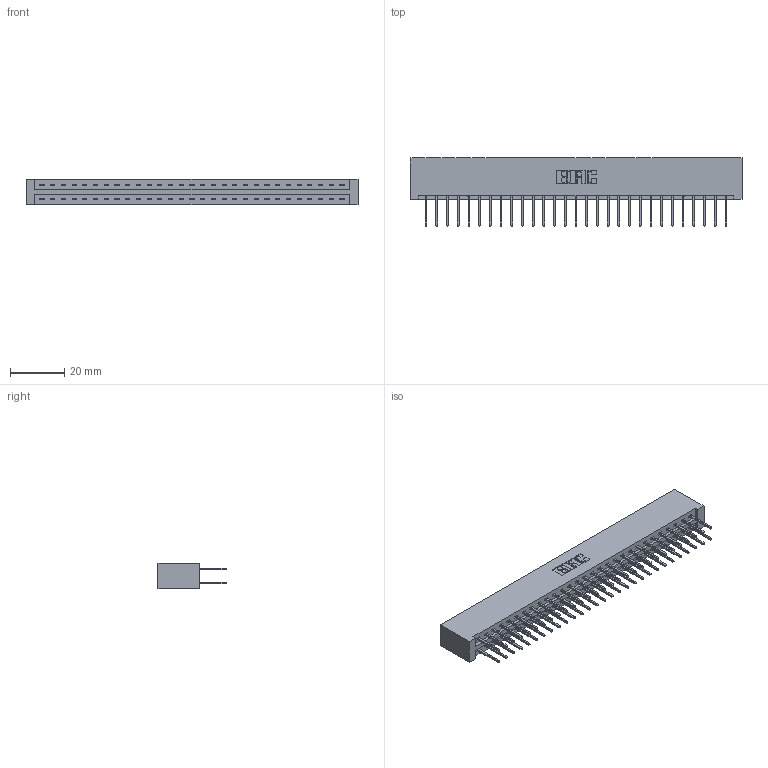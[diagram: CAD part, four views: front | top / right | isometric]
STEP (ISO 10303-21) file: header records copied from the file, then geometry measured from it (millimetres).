
FILE_DESCRIPTION (( 'STEP AP203' ), '1' );
FILE_NAME ('387-058-523-201.STEP', '2019-10-19T08:37:09', ( '' ), ( '' ), 'SwSTEP 2.0', 'SolidWorks 2016', '' );
FILE_SCHEMA (( 'CONFIG_CONTROL_DESIGN' ));
Length unit declared in the file: inch
Products named in the file (3): 387-058-523-201; 337 Part_No Mounting Lugs; 345-292-001_345-293-123
Assembly tree (59 placements, depth 2):
  387-058-523-201
    337 Part_No Mounting Lugs
    345-292-001_345-293-123  x58
Bounding box: 122.78 x 25.15 x 9.4 mm (x, y, z)
Volume: 13646.5 mm3; surface area: 15922.2 mm2
Topology: 59 solids, 59 shells, 3238 faces, 9625 edges, 6338 vertices
Faces by surface type: plane 2270, cylinder 968
Entity records: 23907 total; most frequent: CARTESIAN_POINT 4038, ORIENTED_EDGE 3974, DIRECTION 3451, EDGE_CURVE 1987, VECTOR 1867, LINE 1867, VERTEX_POINT 1322, AXIS2_PLACEMENT_3D 792
